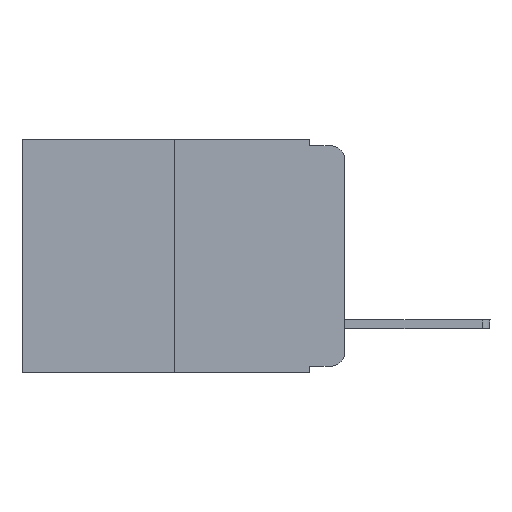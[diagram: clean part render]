
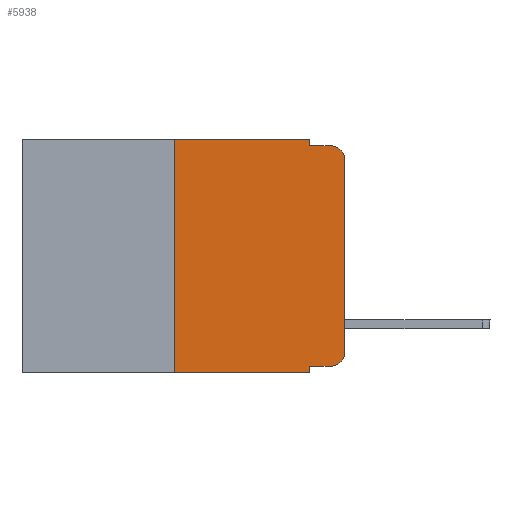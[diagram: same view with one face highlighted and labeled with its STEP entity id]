
A CAD part, left-side view. The second image highlights one B-rep face of the part: STEP entity #5938.
In plain terms, the highlighted planar face has unit normal (-1, 0, 0).
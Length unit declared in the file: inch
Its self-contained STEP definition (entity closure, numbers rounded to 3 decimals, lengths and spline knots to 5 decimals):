
#86 = CARTESIAN_POINT ( 'NONE',  ( 0., 0.473, 0. ) ) ;
#429 = CARTESIAN_POINT ( 'NONE',  ( 0., 0.02, -0.03 ) ) ;
#512 = CARTESIAN_POINT ( 'NONE',  ( 0., 0.051, 0. ) ) ;
#526 = EDGE_CURVE ( 'NONE', #2965, #6741, #6136, .T. ) ;
#543 = DIRECTION ( 'NONE',  ( 0., 0., -1. ) ) ;
#723 = ORIENTED_EDGE ( 'NONE', *, *, #11525, .F. ) ;
#1002 = FACE_OUTER_BOUND ( 'NONE', #2403, .T. ) ;
#1246 = CARTESIAN_POINT ( 'NONE',  ( 0., 0.051, -0.01 ) ) ;
#1276 = DIRECTION ( 'NONE',  ( -1., 0., 0. ) ) ;
#1278 = VECTOR ( 'NONE', #5710, 39.37008 ) ;
#1279 = LINE ( 'NONE', #7673, #9826 ) ;
#1427 = VECTOR ( 'NONE', #4627, 39.37008 ) ;
#1777 = DIRECTION ( 'NONE',  ( -1., 0., 0. ) ) ;
#1890 = EDGE_CURVE ( 'NONE', #10484, #11472, #3262, .T. ) ;
#1902 = ORIENTED_EDGE ( 'NONE', *, *, #5734, .F. ) ;
#2075 = CARTESIAN_POINT ( 'NONE',  ( 0., 0.051, 0. ) ) ;
#2172 = CARTESIAN_POINT ( 'NONE',  ( 0., 0.25, -0.343 ) ) ;
#2403 = EDGE_LOOP ( 'NONE', ( #9607, #7230, #1902, #2483, #4324, #723, #7674, #11002, #5964, #11492 ) ) ;
#2483 = ORIENTED_EDGE ( 'NONE', *, *, #11495, .F. ) ;
#2924 = LINE ( 'NONE', #3820, #9020 ) ;
#2965 = VERTEX_POINT ( 'NONE', #4976 ) ;
#2987 = CARTESIAN_POINT ( 'NONE',  ( 0., 0.051, -0.343 ) ) ;
#3194 = LINE ( 'NONE', #5880, #4904 ) ;
#3262 = CIRCLE ( 'NONE', #10474, 0.02 ) ;
#3611 = LINE ( 'NONE', #10843, #5133 ) ;
#3756 = DIRECTION ( 'NONE',  ( 1., 0., 0. ) ) ;
#3819 = VERTEX_POINT ( 'NONE', #5005 ) ;
#3820 = CARTESIAN_POINT ( 'NONE',  ( 0., 0., 0. ) ) ;
#4063 = EDGE_CURVE ( 'NONE', #5756, #6741, #6479, .T. ) ;
#4151 = DIRECTION ( 'NONE',  ( 0., -1., 0. ) ) ;
#4324 = ORIENTED_EDGE ( 'NONE', *, *, #6092, .F. ) ;
#4627 = DIRECTION ( 'NONE',  ( 0., -1., 0. ) ) ;
#4867 = CARTESIAN_POINT ( 'NONE',  ( 0., 0.02, -0.333 ) ) ;
#4904 = VECTOR ( 'NONE', #4151, 39.37008 ) ;
#4976 = CARTESIAN_POINT ( 'NONE',  ( 0., 0.051, -0.333 ) ) ;
#5005 = CARTESIAN_POINT ( 'NONE',  ( 0., 0., -0.03 ) ) ;
#5133 = VECTOR ( 'NONE', #8069, 39.37008 ) ;
#5710 = DIRECTION ( 'NONE',  ( 0., 0., -1. ) ) ;
#5734 = EDGE_CURVE ( 'NONE', #8273, #11660, #9266, .T. ) ;
#5756 = VERTEX_POINT ( 'NONE', #2172 ) ;
#5862 = EDGE_CURVE ( 'NONE', #11472, #3819, #2924, .T. ) ;
#5880 = CARTESIAN_POINT ( 'NONE',  ( 0., 0.051, -0.333 ) ) ;
#5938 = ADVANCED_FACE ( 'NONE', ( #1002 ), #8272, .F. ) ;
#5964 = ORIENTED_EDGE ( 'NONE', *, *, #10248, .T. ) ;
#6032 = EDGE_CURVE ( 'NONE', #3819, #11660, #7377, .T. ) ;
#6092 = EDGE_CURVE ( 'NONE', #6390, #6892, #3611, .T. ) ;
#6136 = LINE ( 'NONE', #6977, #8326 ) ;
#6390 = VERTEX_POINT ( 'NONE', #6895 ) ;
#6479 = LINE ( 'NONE', #9903, #7810 ) ;
#6538 = DIRECTION ( 'NONE',  ( 0., -1., 0. ) ) ;
#6603 = LINE ( 'NONE', #2075, #1278 ) ;
#6741 = VERTEX_POINT ( 'NONE', #2987 ) ;
#6829 = AXIS2_PLACEMENT_3D ( 'NONE', #429, #1276, #543 ) ;
#6892 = VERTEX_POINT ( 'NONE', #512 ) ;
#6895 = CARTESIAN_POINT ( 'NONE',  ( 0., 0.25, 0. ) ) ;
#6977 = CARTESIAN_POINT ( 'NONE',  ( 0., 0.051, 0. ) ) ;
#7230 = ORIENTED_EDGE ( 'NONE', *, *, #6032, .T. ) ;
#7306 = CARTESIAN_POINT ( 'NONE',  ( 0., 0.051, -0.01 ) ) ;
#7377 = CIRCLE ( 'NONE', #6829, 0.02 ) ;
#7395 = DIRECTION ( 'NONE',  ( 0., 0., -1. ) ) ;
#7673 = CARTESIAN_POINT ( 'NONE',  ( 0., 0.25, 0. ) ) ;
#7674 = ORIENTED_EDGE ( 'NONE', *, *, #4063, .T. ) ;
#7810 = VECTOR ( 'NONE', #6538, 39.37008 ) ;
#8069 = DIRECTION ( 'NONE',  ( 0., -1., 0. ) ) ;
#8139 = DIRECTION ( 'NONE',  ( 0., 0., -1. ) ) ;
#8221 = DIRECTION ( 'NONE',  ( 0., 0., 1. ) ) ;
#8272 = PLANE ( 'NONE',  #8852 ) ;
#8273 = VERTEX_POINT ( 'NONE', #1246 ) ;
#8326 = VECTOR ( 'NONE', #8844, 39.37008 ) ;
#8482 = DIRECTION ( 'NONE',  ( 0., 0., 1. ) ) ;
#8844 = DIRECTION ( 'NONE',  ( 0., 0., -1. ) ) ;
#8852 = AXIS2_PLACEMENT_3D ( 'NONE', #86, #3756, #7395 ) ;
#9020 = VECTOR ( 'NONE', #8221, 39.37008 ) ;
#9266 = LINE ( 'NONE', #7306, #1427 ) ;
#9607 = ORIENTED_EDGE ( 'NONE', *, *, #5862, .T. ) ;
#9826 = VECTOR ( 'NONE', #8482, 39.37008 ) ;
#9903 = CARTESIAN_POINT ( 'NONE',  ( 0., 0.473, -0.343 ) ) ;
#9906 = CARTESIAN_POINT ( 'NONE',  ( 0., 0.02, -0.313 ) ) ;
#10248 = EDGE_CURVE ( 'NONE', #2965, #10484, #3194, .T. ) ;
#10474 = AXIS2_PLACEMENT_3D ( 'NONE', #9906, #1777, #8139 ) ;
#10484 = VERTEX_POINT ( 'NONE', #4867 ) ;
#10689 = CARTESIAN_POINT ( 'NONE',  ( 0., 0.02, -0.01 ) ) ;
#10843 = CARTESIAN_POINT ( 'NONE',  ( 0., 0.473, 0. ) ) ;
#11002 = ORIENTED_EDGE ( 'NONE', *, *, #526, .F. ) ;
#11082 = CARTESIAN_POINT ( 'NONE',  ( 0., 0., -0.313 ) ) ;
#11472 = VERTEX_POINT ( 'NONE', #11082 ) ;
#11492 = ORIENTED_EDGE ( 'NONE', *, *, #1890, .T. ) ;
#11495 = EDGE_CURVE ( 'NONE', #6892, #8273, #6603, .T. ) ;
#11525 = EDGE_CURVE ( 'NONE', #5756, #6390, #1279, .T. ) ;
#11660 = VERTEX_POINT ( 'NONE', #10689 ) ;
